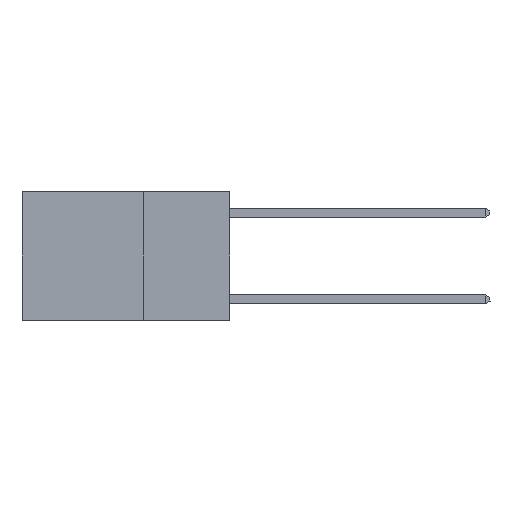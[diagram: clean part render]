
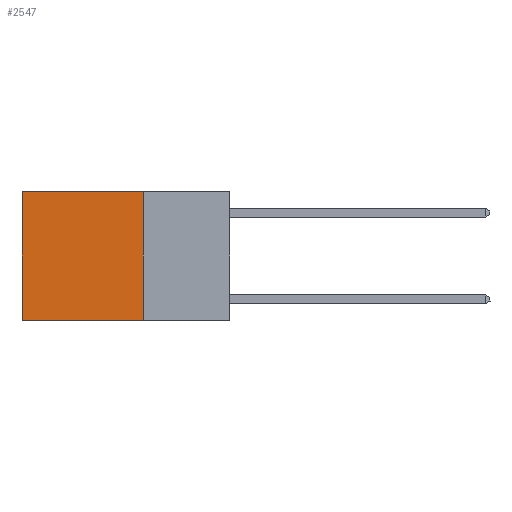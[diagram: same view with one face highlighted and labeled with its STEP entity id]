
A CAD part, left-side view. The second image highlights one B-rep face of the part: STEP entity #2547.
In plain terms, the highlighted planar face has unit normal (-1, 0, 0).
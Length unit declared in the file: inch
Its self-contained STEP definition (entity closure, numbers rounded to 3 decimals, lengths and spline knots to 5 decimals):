
#173 = LINE ( 'NONE', #4320, #2454 ) ;
#350 = CARTESIAN_POINT ( 'NONE',  ( 0.2625, 0.25, 0. ) ) ;
#405 = EDGE_CURVE ( 'NONE', #9910, #10975, #173, .T. ) ;
#1039 = LINE ( 'NONE', #5782, #2550 ) ;
#1610 = CARTESIAN_POINT ( 'NONE',  ( 0.2625, 0.6, 0. ) ) ;
#1732 = PLANE ( 'NONE',  #2051 ) ;
#2051 = AXIS2_PLACEMENT_3D ( 'NONE', #9675, #7839, #2324 ) ;
#2072 = LINE ( 'NONE', #3949, #11218 ) ;
#2181 = EDGE_CURVE ( 'NONE', #9910, #10905, #2072, .T. ) ;
#2324 = DIRECTION ( 'NONE',  ( 0., 0., -1. ) ) ;
#2454 = VECTOR ( 'NONE', #7352, 39.37008 ) ;
#2547 = ADVANCED_FACE ( 'NONE', ( #4187 ), #1732, .F. ) ;
#2550 = VECTOR ( 'NONE', #5826, 39.37008 ) ;
#3717 = ORIENTED_EDGE ( 'NONE', *, *, #9235, .T. ) ;
#3949 = CARTESIAN_POINT ( 'NONE',  ( 0.2625, 0.25, 0. ) ) ;
#4187 = FACE_OUTER_BOUND ( 'NONE', #8333, .T. ) ;
#4320 = CARTESIAN_POINT ( 'NONE',  ( 0.2625, 0.25, 0. ) ) ;
#5371 = VECTOR ( 'NONE', #12352, 39.37008 ) ;
#5782 = CARTESIAN_POINT ( 'NONE',  ( 0.2625, 0.6, 0. ) ) ;
#5826 = DIRECTION ( 'NONE',  ( 0., 0., -1. ) ) ;
#7144 = ORIENTED_EDGE ( 'NONE', *, *, #11000, .F. ) ;
#7352 = DIRECTION ( 'NONE',  ( 0., 0., -1. ) ) ;
#7587 = CARTESIAN_POINT ( 'NONE',  ( 0.2625, 0.25, -0.37 ) ) ;
#7839 = DIRECTION ( 'NONE',  ( 1., 0., 0. ) ) ;
#8333 = EDGE_LOOP ( 'NONE', ( #3717, #7144, #11238, #9852 ) ) ;
#8555 = CARTESIAN_POINT ( 'NONE',  ( 0.2625, 0.25, -0.37 ) ) ;
#8670 = DIRECTION ( 'NONE',  ( 0., 1., 0. ) ) ;
#9235 = EDGE_CURVE ( 'NONE', #10905, #10671, #1039, .T. ) ;
#9675 = CARTESIAN_POINT ( 'NONE',  ( 0.2625, 0.25, 0. ) ) ;
#9852 = ORIENTED_EDGE ( 'NONE', *, *, #2181, .T. ) ;
#9910 = VERTEX_POINT ( 'NONE', #350 ) ;
#10671 = VERTEX_POINT ( 'NONE', #10992 ) ;
#10905 = VERTEX_POINT ( 'NONE', #1610 ) ;
#10975 = VERTEX_POINT ( 'NONE', #7587 ) ;
#10992 = CARTESIAN_POINT ( 'NONE',  ( 0.2625, 0.6, -0.37 ) ) ;
#11000 = EDGE_CURVE ( 'NONE', #10975, #10671, #11035, .T. ) ;
#11035 = LINE ( 'NONE', #8555, #5371 ) ;
#11218 = VECTOR ( 'NONE', #8670, 39.37008 ) ;
#11238 = ORIENTED_EDGE ( 'NONE', *, *, #405, .F. ) ;
#12352 = DIRECTION ( 'NONE',  ( 0., 1., 0. ) ) ;
